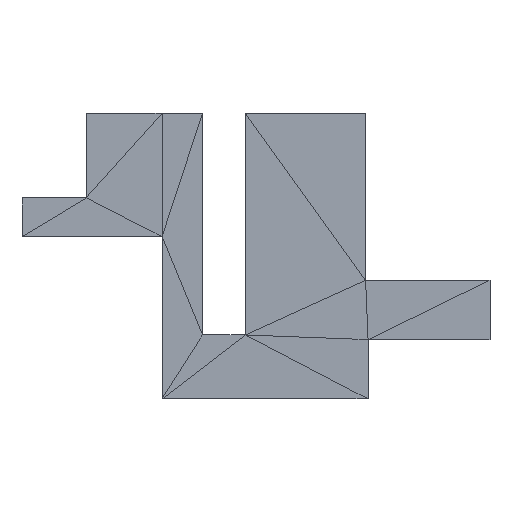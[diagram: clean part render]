
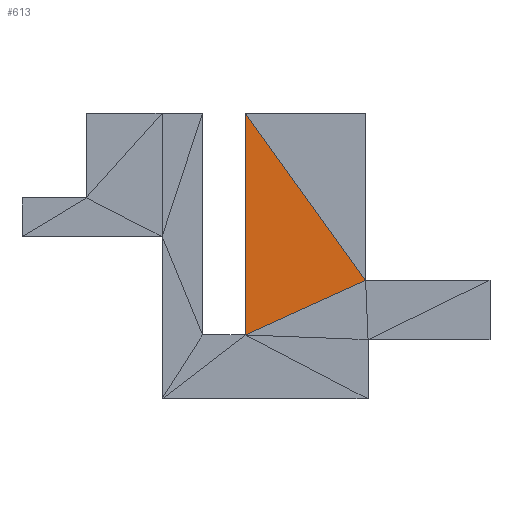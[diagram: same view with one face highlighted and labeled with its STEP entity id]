
A CAD part, top view. The second image highlights one B-rep face of the part: STEP entity #613.
In plain terms, the highlighted planar face has unit normal (0, 0, 1).
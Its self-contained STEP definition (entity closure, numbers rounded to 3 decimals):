
#281 = VERTEX_POINT('',#282);
#282 = CARTESIAN_POINT('',(3.303,-11.986,6.097
    ));
#513 = VERTEX_POINT('',#514);
#514 = CARTESIAN_POINT('',(21.844,-3.556,
    6.097));
#528 = PLANE('',#529);
#529 = AXIS2_PLACEMENT_3D('',#530,#531,#532);
#530 = CARTESIAN_POINT('',(14.435,-9.624,
    6.097));
#531 = DIRECTION('',(0.,0.,1.));
#532 = DIRECTION('',(0.,1.,0.));
#589 = EDGE_CURVE('',#513,#281,#590,.T.);
#590 = SURFACE_CURVE('',#591,(#595,#602),.PCURVE_S1.);
#591 = LINE('',#592,#593);
#592 = CARTESIAN_POINT('',(21.844,-3.556,
    6.097));
#593 = VECTOR('',#594,1.);
#594 = DIRECTION('',(-0.91,-0.414,0.));
#595 = PCURVE('',#528,#596);
#596 = DEFINITIONAL_REPRESENTATION('',(#597),#601);
#597 = LINE('',#598,#599);
#598 = CARTESIAN_POINT('',(6.068,-7.409));
#599 = VECTOR('',#600,1.);
#600 = DIRECTION('',(-0.414,0.91));
#601 = ( GEOMETRIC_REPRESENTATION_CONTEXT(2) 
PARAMETRIC_REPRESENTATION_CONTEXT() REPRESENTATION_CONTEXT('2D SPACE',''
  ) );
#602 = PCURVE('',#603,#608);
#603 = PLANE('',#604);
#604 = AXIS2_PLACEMENT_3D('',#605,#606,#607);
#605 = CARTESIAN_POINT('',(8.9,3.629,6.097)
  );
#606 = DIRECTION('',(0.,0.,1.));
#607 = DIRECTION('',(1.,0.,0.));
#608 = DEFINITIONAL_REPRESENTATION('',(#609),#612);
#609 = B_SPLINE_CURVE_WITH_KNOTS('',1,(#610,#611),.UNSPECIFIED.,.F.,.F.,
  (2,2),(0.,20.367),.PIECEWISE_BEZIER_KNOTS.);
#610 = CARTESIAN_POINT('',(12.944,-7.185));
#611 = CARTESIAN_POINT('',(-5.597,-15.615));
#612 = ( GEOMETRIC_REPRESENTATION_CONTEXT(2) 
PARAMETRIC_REPRESENTATION_CONTEXT() REPRESENTATION_CONTEXT('2D SPACE',''
  ) );
#613 = ADVANCED_FACE('',(#614),#603,.T.);
#614 = FACE_BOUND('',#615,.T.);
#615 = EDGE_LOOP('',(#616,#617,#644));
#616 = ORIENTED_EDGE('',*,*,#589,.F.);
#617 = ORIENTED_EDGE('',*,*,#618,.F.);
#618 = EDGE_CURVE('',#619,#513,#621,.T.);
#619 = VERTEX_POINT('',#620);
#620 = CARTESIAN_POINT('',(3.303,22.225,6.097)
  );
#621 = SURFACE_CURVE('',#622,(#626,#632),.PCURVE_S1.);
#622 = LINE('',#623,#624);
#623 = CARTESIAN_POINT('',(3.303,22.225,6.097)
  );
#624 = VECTOR('',#625,1.);
#625 = DIRECTION('',(0.584,-0.812,0.));
#626 = PCURVE('',#603,#627);
#627 = DEFINITIONAL_REPRESENTATION('',(#628),#631);
#628 = B_SPLINE_CURVE_WITH_KNOTS('',1,(#629,#630),.UNSPECIFIED.,.F.,.F.,
  (2,2),(0.,31.756),.PIECEWISE_BEZIER_KNOTS.);
#629 = CARTESIAN_POINT('',(-5.597,18.596));
#630 = CARTESIAN_POINT('',(12.944,-7.185));
#631 = ( GEOMETRIC_REPRESENTATION_CONTEXT(2) 
PARAMETRIC_REPRESENTATION_CONTEXT() REPRESENTATION_CONTEXT('2D SPACE',''
  ) );
#632 = PCURVE('',#633,#638);
#633 = PLANE('',#634);
#634 = AXIS2_PLACEMENT_3D('',#635,#636,#637);
#635 = CARTESIAN_POINT('',(15.715,12.476,
    6.097));
#636 = DIRECTION('',(0.,0.,1.));
#637 = DIRECTION('',(1.,0.,-0.));
#638 = DEFINITIONAL_REPRESENTATION('',(#639),#643);
#639 = LINE('',#640,#641);
#640 = CARTESIAN_POINT('',(-12.412,9.749));
#641 = VECTOR('',#642,1.);
#642 = DIRECTION('',(0.584,-0.812));
#643 = ( GEOMETRIC_REPRESENTATION_CONTEXT(2) 
PARAMETRIC_REPRESENTATION_CONTEXT() REPRESENTATION_CONTEXT('2D SPACE',''
  ) );
#644 = ORIENTED_EDGE('',*,*,#645,.T.);
#645 = EDGE_CURVE('',#619,#281,#646,.T.);
#646 = SURFACE_CURVE('',#647,(#651,#658),.PCURVE_S1.);
#647 = LINE('',#648,#649);
#648 = CARTESIAN_POINT('',(3.303,22.225,6.097)
  );
#649 = VECTOR('',#650,1.);
#650 = DIRECTION('',(0.,-1.,0.));
#651 = PCURVE('',#603,#652);
#652 = DEFINITIONAL_REPRESENTATION('',(#653),#657);
#653 = LINE('',#654,#655);
#654 = CARTESIAN_POINT('',(-5.597,18.596));
#655 = VECTOR('',#656,1.);
#656 = DIRECTION('',(0.,-1.));
#657 = ( GEOMETRIC_REPRESENTATION_CONTEXT(2) 
PARAMETRIC_REPRESENTATION_CONTEXT() REPRESENTATION_CONTEXT('2D SPACE',''
  ) );
#658 = PCURVE('',#659,#664);
#659 = PLANE('',#660);
#660 = AXIS2_PLACEMENT_3D('',#661,#662,#663);
#661 = CARTESIAN_POINT('',(3.303,3.73,4.438)
  );
#662 = DIRECTION('',(-1.,-0.,-0.));
#663 = DIRECTION('',(0.,0.,-1.));
#664 = DEFINITIONAL_REPRESENTATION('',(#665),#668);
#665 = B_SPLINE_CURVE_WITH_KNOTS('',1,(#666,#667),.UNSPECIFIED.,.F.,.F.,
  (2,2),(0.,34.211),.PIECEWISE_BEZIER_KNOTS.);
#666 = CARTESIAN_POINT('',(-1.659,-18.495));
#667 = CARTESIAN_POINT('',(-1.659,15.716));
#668 = ( GEOMETRIC_REPRESENTATION_CONTEXT(2) 
PARAMETRIC_REPRESENTATION_CONTEXT() REPRESENTATION_CONTEXT('2D SPACE',''
  ) );
